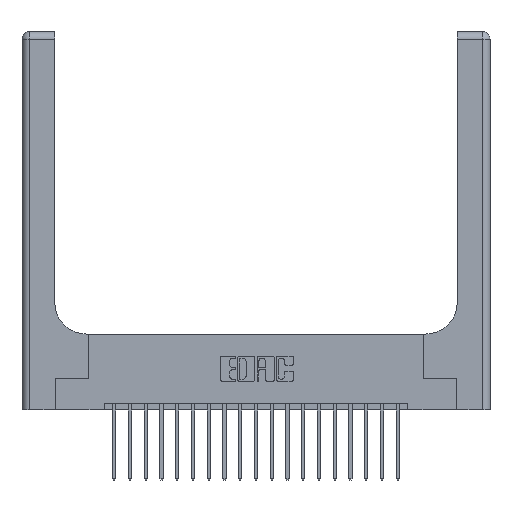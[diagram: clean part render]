
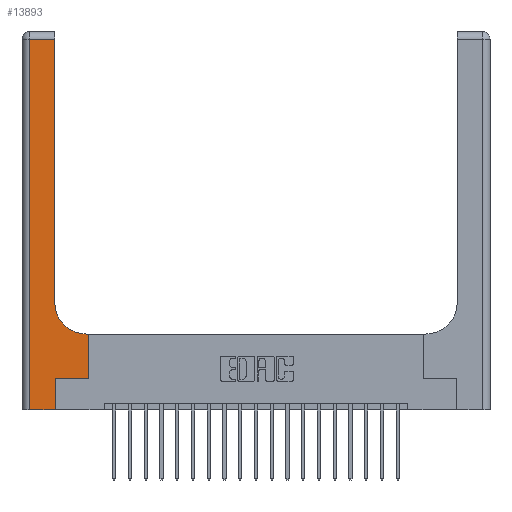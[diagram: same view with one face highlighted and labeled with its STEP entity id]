
A CAD part, top view. The second image highlights one B-rep face of the part: STEP entity #13893.
In plain terms, the highlighted planar face has unit normal (0, 0, 1).
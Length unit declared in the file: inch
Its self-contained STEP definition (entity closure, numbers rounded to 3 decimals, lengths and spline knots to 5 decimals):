
#224 = LINE ( 'NONE', #8942, #17274 ) ;
#270 = EDGE_CURVE ( 'NONE', #17872, #6645, #7726, .T. ) ;
#1001 = CARTESIAN_POINT ( 'NONE',  ( 0.51, 0.85, 0.37 ) ) ;
#1123 = CARTESIAN_POINT ( 'NONE',  ( 0.265, 0.25, 0.37 ) ) ;
#1682 = ORIENTED_EDGE ( 'NONE', *, *, #7813, .T. ) ;
#2173 = CARTESIAN_POINT ( 'NONE',  ( 0.528, 0.25, 0.37 ) ) ;
#2241 = VERTEX_POINT ( 'NONE', #19999 ) ;
#2248 = DIRECTION ( 'NONE',  ( 0., 1., 0. ) ) ;
#2390 = VERTEX_POINT ( 'NONE', #3176 ) ;
#3176 = CARTESIAN_POINT ( 'NONE',  ( 0.265, 0., 0.37 ) ) ;
#3546 = LINE ( 'NONE', #18230, #16056 ) ;
#4062 = CARTESIAN_POINT ( 'NONE',  ( 0.06, 2.94, 0.37 ) ) ;
#4082 = DIRECTION ( 'NONE',  ( 0., 0., -1. ) ) ;
#4109 = VERTEX_POINT ( 'NONE', #7780 ) ;
#4445 = ORIENTED_EDGE ( 'NONE', *, *, #16229, .T. ) ;
#4751 = DIRECTION ( 'NONE',  ( -1., 0., 0. ) ) ;
#4811 = VECTOR ( 'NONE', #4751, 39.37008 ) ;
#5048 = ORIENTED_EDGE ( 'NONE', *, *, #20312, .T. ) ;
#5169 = VECTOR ( 'NONE', #18611, 39.37008 ) ;
#5184 = VERTEX_POINT ( 'NONE', #12983 ) ;
#5410 = FACE_OUTER_BOUND ( 'NONE', #7917, .T. ) ;
#5642 = CARTESIAN_POINT ( 'NONE',  ( 0.06, 0., 0.37 ) ) ;
#6052 = VECTOR ( 'NONE', #13157, 39.37008 ) ;
#6084 = LINE ( 'NONE', #8932, #12615 ) ;
#6477 = EDGE_CURVE ( 'NONE', #15236, #2241, #7002, .T. ) ;
#6645 = VERTEX_POINT ( 'NONE', #5642 ) ;
#6737 = VECTOR ( 'NONE', #2248, 39.37008 ) ;
#7002 = LINE ( 'NONE', #2173, #6737 ) ;
#7297 = PLANE ( 'NONE',  #14937 ) ;
#7610 = CARTESIAN_POINT ( 'NONE',  ( 0.06, 3., 0.37 ) ) ;
#7726 = LINE ( 'NONE', #7610, #14008 ) ;
#7776 = VERTEX_POINT ( 'NONE', #9656 ) ;
#7780 = CARTESIAN_POINT ( 'NONE',  ( 0.26, 2.94, 0.37 ) ) ;
#7813 = EDGE_CURVE ( 'NONE', #2390, #9281, #12583, .T. ) ;
#7917 = EDGE_LOOP ( 'NONE', ( #17087, #4445, #15078, #18237, #1682, #5048, #9953, #8844, #10540 ) ) ;
#8844 = ORIENTED_EDGE ( 'NONE', *, *, #17059, .T. ) ;
#8932 = CARTESIAN_POINT ( 'NONE',  ( 0.26, 3., 0.37 ) ) ;
#8942 = CARTESIAN_POINT ( 'NONE',  ( 0., 0., 0.37 ) ) ;
#9281 = VERTEX_POINT ( 'NONE', #15500 ) ;
#9656 = CARTESIAN_POINT ( 'NONE',  ( 0.51, 0.6, 0.37 ) ) ;
#9953 = ORIENTED_EDGE ( 'NONE', *, *, #6477, .T. ) ;
#10165 = CARTESIAN_POINT ( 'NONE',  ( 0.528, 0.25, 0.37 ) ) ;
#10503 = EDGE_CURVE ( 'NONE', #7776, #5184, #15467, .T. ) ;
#10540 = ORIENTED_EDGE ( 'NONE', *, *, #10503, .T. ) ;
#12093 = DIRECTION ( 'NONE',  ( 0., -1., 0. ) ) ;
#12255 = DIRECTION ( 'NONE',  ( 0., 0., -1. ) ) ;
#12583 = LINE ( 'NONE', #19521, #6052 ) ;
#12615 = VECTOR ( 'NONE', #15094, 39.37008 ) ;
#12983 = CARTESIAN_POINT ( 'NONE',  ( 0.26, 0.85, 0.37 ) ) ;
#13157 = DIRECTION ( 'NONE',  ( 0., 1., 0. ) ) ;
#13564 = CARTESIAN_POINT ( 'NONE',  ( 0., 3., 0.37 ) ) ;
#13729 = LINE ( 'NONE', #1123, #5169 ) ;
#13893 = ADVANCED_FACE ( 'NONE', ( #5410 ), #7297, .F. ) ;
#14008 = VECTOR ( 'NONE', #12093, 39.37008 ) ;
#14937 = AXIS2_PLACEMENT_3D ( 'NONE', #13564, #4082, #18500 ) ;
#15078 = ORIENTED_EDGE ( 'NONE', *, *, #270, .T. ) ;
#15094 = DIRECTION ( 'NONE',  ( 0., 1., 0. ) ) ;
#15098 = DIRECTION ( 'NONE',  ( -1., 0., 0. ) ) ;
#15236 = VERTEX_POINT ( 'NONE', #10165 ) ;
#15357 = EDGE_CURVE ( 'NONE', #5184, #4109, #6084, .T. ) ;
#15467 = CIRCLE ( 'NONE', #20273, 0.25 ) ;
#15500 = CARTESIAN_POINT ( 'NONE',  ( 0.265, 0.25, 0.37 ) ) ;
#16056 = VECTOR ( 'NONE', #15098, 39.37008 ) ;
#16229 = EDGE_CURVE ( 'NONE', #4109, #17872, #18355, .T. ) ;
#16916 = DIRECTION ( 'NONE',  ( 1., 0., 0. ) ) ;
#17059 = EDGE_CURVE ( 'NONE', #2241, #7776, #3546, .T. ) ;
#17087 = ORIENTED_EDGE ( 'NONE', *, *, #15357, .T. ) ;
#17274 = VECTOR ( 'NONE', #16916, 39.37008 ) ;
#17872 = VERTEX_POINT ( 'NONE', #4062 ) ;
#18230 = CARTESIAN_POINT ( 'NONE',  ( 0.26, 0.6, 0.37 ) ) ;
#18237 = ORIENTED_EDGE ( 'NONE', *, *, #19111, .T. ) ;
#18355 = LINE ( 'NONE', #20690, #4811 ) ;
#18500 = DIRECTION ( 'NONE',  ( -1., 0., 0. ) ) ;
#18611 = DIRECTION ( 'NONE',  ( 1., 0., 0. ) ) ;
#18754 = DIRECTION ( 'NONE',  ( 1., 0., 0. ) ) ;
#19111 = EDGE_CURVE ( 'NONE', #6645, #2390, #224, .T. ) ;
#19521 = CARTESIAN_POINT ( 'NONE',  ( 0.265, 0., 0.37 ) ) ;
#19999 = CARTESIAN_POINT ( 'NONE',  ( 0.528, 0.6, 0.37 ) ) ;
#20273 = AXIS2_PLACEMENT_3D ( 'NONE', #1001, #12255, #18754 ) ;
#20312 = EDGE_CURVE ( 'NONE', #9281, #15236, #13729, .T. ) ;
#20690 = CARTESIAN_POINT ( 'NONE',  ( 0., 2.94, 0.37 ) ) ;
